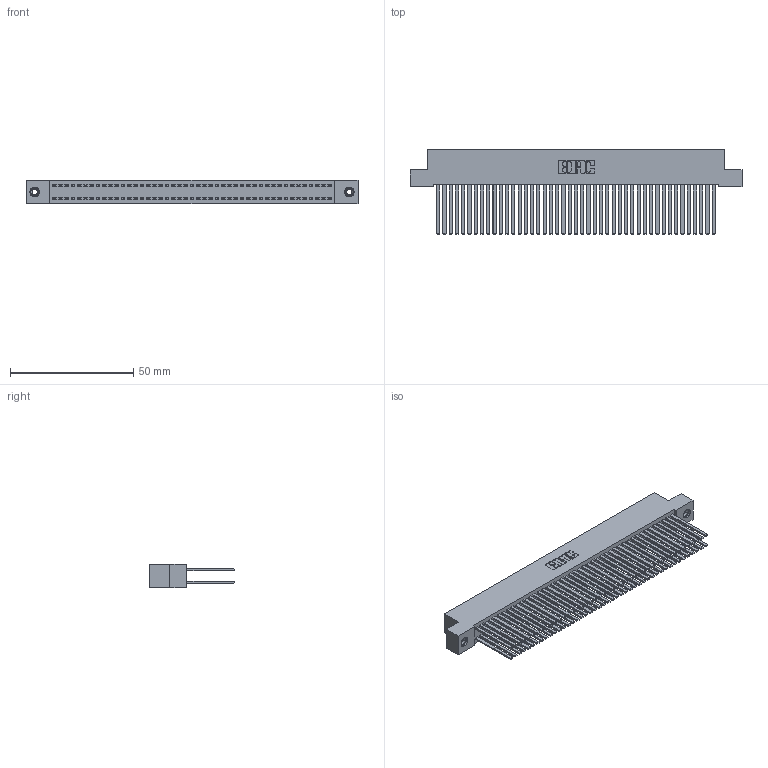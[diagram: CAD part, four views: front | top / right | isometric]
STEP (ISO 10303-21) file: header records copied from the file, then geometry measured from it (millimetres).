
FILE_DESCRIPTION (( 'STEP AP203' ), '1' );
FILE_NAME ('392-090-544-208.STEP', '2018-08-18T07:13:45', ( '' ), ( '' ), 'SwSTEP 2.0', 'SolidWorks 2016', '' );
FILE_SCHEMA (( 'CONFIG_CONTROL_DESIGN' ));
Length unit declared in the file: inch
Products named in the file (4): 342 Part_TI; 345-292-001_345-293-144; 345-250-001_345-250-003-102; 392-090-544-208
Assembly tree (93 placements, depth 2):
  392-090-544-208
    342 Part_TI
    345-292-001_345-293-144  x90
    345-250-001_345-250-003-102  x2
Bounding box: 134.62 x 34.3 x 9.4 mm (x, y, z)
Volume: 13365.7 mm3; surface area: 25334.2 mm2
Topology: 93 solids, 93 shells, 4310 faces, 12765 edges, 8382 vertices
Faces by surface type: plane 2978, cylinder 1316, cone 12, torus 4
Entity records: 29432 total; most frequent: CARTESIAN_POINT 4853, ORIENTED_EDGE 4782, DIRECTION 4169, EDGE_CURVE 2391, LINE 2247, VECTOR 2247, VERTEX_POINT 1588, AXIS2_PLACEMENT_3D 961
